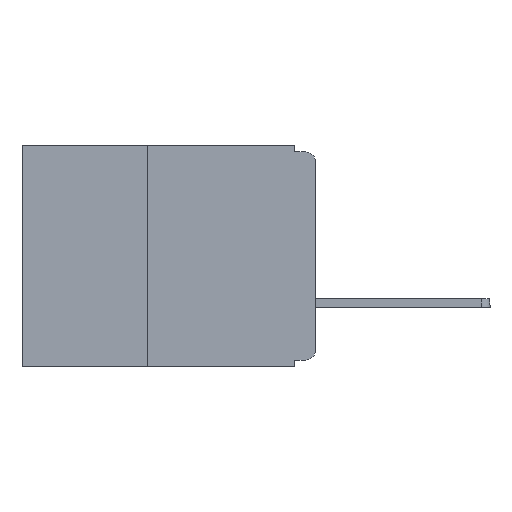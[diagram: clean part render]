
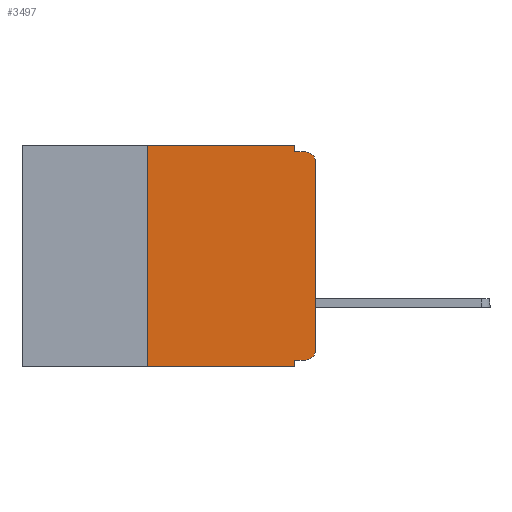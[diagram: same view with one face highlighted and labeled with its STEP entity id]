
A CAD part, left-side view. The second image highlights one B-rep face of the part: STEP entity #3497.
In plain terms, the highlighted planar face has unit normal (-1, 0, 0).
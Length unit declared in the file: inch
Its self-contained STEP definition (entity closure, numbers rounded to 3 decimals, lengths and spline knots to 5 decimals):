
#154 = VECTOR ( 'NONE', #29378, 39.37008 ) ;
#1849 = ORIENTED_EDGE ( 'NONE', *, *, #22647, .T. ) ;
#2197 = ORIENTED_EDGE ( 'NONE', *, *, #25418, .F. ) ;
#2333 = DIRECTION ( 'NONE',  ( 0., 1., 0. ) ) ;
#2856 = VECTOR ( 'NONE', #24973, 39.37008 ) ;
#2929 = CARTESIAN_POINT ( 'NONE',  ( 0., 0.015, -0.32 ) ) ;
#3090 = CARTESIAN_POINT ( 'NONE',  ( 0., 0., -0.32 ) ) ;
#3497 = ADVANCED_FACE ( 'NONE', ( #12537 ), #16946, .F. ) ;
#3577 = CARTESIAN_POINT ( 'NONE',  ( 0., 0.031, -0.33 ) ) ;
#3634 = DIRECTION ( 'NONE',  ( 0., 0., -1. ) ) ;
#3754 = CARTESIAN_POINT ( 'NONE',  ( 0., 0.25, -0.33 ) ) ;
#3761 = EDGE_CURVE ( 'NONE', #8588, #11195, #12156, .T. ) ;
#4030 = ORIENTED_EDGE ( 'NONE', *, *, #3761, .F. ) ;
#4034 = DIRECTION ( 'NONE',  ( 0., 0., -1. ) ) ;
#4090 = DIRECTION ( 'NONE',  ( -1., 0., 0. ) ) ;
#4236 = CARTESIAN_POINT ( 'NONE',  ( 0., 0.015, -0.305 ) ) ;
#4322 = LINE ( 'NONE', #6348, #2856 ) ;
#4365 = EDGE_CURVE ( 'NONE', #22120, #13351, #18727, .T. ) ;
#4521 = VECTOR ( 'NONE', #2333, 39.37008 ) ;
#4618 = EDGE_CURVE ( 'NONE', #8588, #7056, #29837, .T. ) ;
#4722 = ORIENTED_EDGE ( 'NONE', *, *, #4365, .T. ) ;
#6168 = CARTESIAN_POINT ( 'NONE',  ( 0., 0.437, -0.33 ) ) ;
#6348 = CARTESIAN_POINT ( 'NONE',  ( 0., 0.437, 0. ) ) ;
#6471 = CARTESIAN_POINT ( 'NONE',  ( 0., 0.031, -0.33 ) ) ;
#6832 = CARTESIAN_POINT ( 'NONE',  ( 0., 0.015, -0.01 ) ) ;
#7056 = VERTEX_POINT ( 'NONE', #10760 ) ;
#7642 = EDGE_CURVE ( 'NONE', #11195, #17058, #18874, .T. ) ;
#7808 = AXIS2_PLACEMENT_3D ( 'NONE', #16616, #16360, #16102 ) ;
#8018 = LINE ( 'NONE', #3754, #14193 ) ;
#8419 = ORIENTED_EDGE ( 'NONE', *, *, #13763, .F. ) ;
#8588 = VERTEX_POINT ( 'NONE', #2929 ) ;
#8792 = DIRECTION ( 'NONE',  ( 0., -1., 0. ) ) ;
#8812 = LINE ( 'NONE', #6168, #14248 ) ;
#9307 = CARTESIAN_POINT ( 'NONE',  ( 0., 0.031, 0. ) ) ;
#9363 = LINE ( 'NONE', #19954, #21024 ) ;
#10125 = DIRECTION ( 'NONE',  ( 0., 0., -1. ) ) ;
#10129 = DIRECTION ( 'NONE',  ( -1., 0., 0. ) ) ;
#10165 = CARTESIAN_POINT ( 'NONE',  ( 0., 0.015, -0.025 ) ) ;
#10760 = CARTESIAN_POINT ( 'NONE',  ( 0., 0., -0.305 ) ) ;
#11113 = CARTESIAN_POINT ( 'NONE',  ( 0., 0., -0.025 ) ) ;
#11195 = VERTEX_POINT ( 'NONE', #21760 ) ;
#11541 = LINE ( 'NONE', #15698, #23219 ) ;
#11611 = CARTESIAN_POINT ( 'NONE',  ( 0., 0.25, 0. ) ) ;
#12028 = EDGE_CURVE ( 'NONE', #18110, #22238, #8018, .T. ) ;
#12156 = LINE ( 'NONE', #3090, #4521 ) ;
#12537 = FACE_OUTER_BOUND ( 'NONE', #16048, .T. ) ;
#12648 = EDGE_CURVE ( 'NONE', #22238, #15921, #4322, .T. ) ;
#12840 = DIRECTION ( 'NONE',  ( 0., 0., -1. ) ) ;
#13267 = VERTEX_POINT ( 'NONE', #29591 ) ;
#13351 = VERTEX_POINT ( 'NONE', #6832 ) ;
#13763 = EDGE_CURVE ( 'NONE', #15921, #13267, #9363, .T. ) ;
#14193 = VECTOR ( 'NONE', #29177, 39.37008 ) ;
#14248 = VECTOR ( 'NONE', #29270, 39.37008 ) ;
#15255 = AXIS2_PLACEMENT_3D ( 'NONE', #4236, #4090, #4034 ) ;
#15698 = CARTESIAN_POINT ( 'NONE',  ( 0., 0., -0.01 ) ) ;
#15853 = AXIS2_PLACEMENT_3D ( 'NONE', #10165, #10129, #10125 ) ;
#15921 = VERTEX_POINT ( 'NONE', #9307 ) ;
#16048 = EDGE_LOOP ( 'NONE', ( #27236, #4722, #2197, #8419, #16064, #17518, #1849, #20441, #4030, #29407 ) ) ;
#16064 = ORIENTED_EDGE ( 'NONE', *, *, #12648, .F. ) ;
#16102 = DIRECTION ( 'NONE',  ( 0., 0., -1. ) ) ;
#16360 = DIRECTION ( 'NONE',  ( 1., 0., 0. ) ) ;
#16616 = CARTESIAN_POINT ( 'NONE',  ( 0., 0.437, 0. ) ) ;
#16680 = VECTOR ( 'NONE', #12840, 39.37008 ) ;
#16946 = PLANE ( 'NONE',  #7808 ) ;
#17058 = VERTEX_POINT ( 'NONE', #6471 ) ;
#17518 = ORIENTED_EDGE ( 'NONE', *, *, #12028, .F. ) ;
#17834 = CARTESIAN_POINT ( 'NONE',  ( 0., 0.25, -0.33 ) ) ;
#18110 = VERTEX_POINT ( 'NONE', #17834 ) ;
#18727 = CIRCLE ( 'NONE', #15853, 0.015 ) ;
#18874 = LINE ( 'NONE', #3577, #16680 ) ;
#19954 = CARTESIAN_POINT ( 'NONE',  ( 0., 0.031, 0. ) ) ;
#20441 = ORIENTED_EDGE ( 'NONE', *, *, #7642, .F. ) ;
#21024 = VECTOR ( 'NONE', #3634, 39.37008 ) ;
#21760 = CARTESIAN_POINT ( 'NONE',  ( 0., 0.031, -0.32 ) ) ;
#22120 = VERTEX_POINT ( 'NONE', #11113 ) ;
#22238 = VERTEX_POINT ( 'NONE', #11611 ) ;
#22647 = EDGE_CURVE ( 'NONE', #18110, #17058, #8812, .T. ) ;
#23219 = VECTOR ( 'NONE', #8792, 39.37008 ) ;
#24900 = LINE ( 'NONE', #27087, #154 ) ;
#24973 = DIRECTION ( 'NONE',  ( 0., -1., 0. ) ) ;
#25418 = EDGE_CURVE ( 'NONE', #13267, #13351, #11541, .T. ) ;
#27087 = CARTESIAN_POINT ( 'NONE',  ( 0., 0., 0. ) ) ;
#27236 = ORIENTED_EDGE ( 'NONE', *, *, #28771, .T. ) ;
#28771 = EDGE_CURVE ( 'NONE', #7056, #22120, #24900, .T. ) ;
#29177 = DIRECTION ( 'NONE',  ( 0., 0., 1. ) ) ;
#29270 = DIRECTION ( 'NONE',  ( 0., -1., 0. ) ) ;
#29378 = DIRECTION ( 'NONE',  ( 0., 0., 1. ) ) ;
#29407 = ORIENTED_EDGE ( 'NONE', *, *, #4618, .T. ) ;
#29591 = CARTESIAN_POINT ( 'NONE',  ( 0., 0.031, -0.01 ) ) ;
#29837 = CIRCLE ( 'NONE', #15255, 0.015 ) ;
